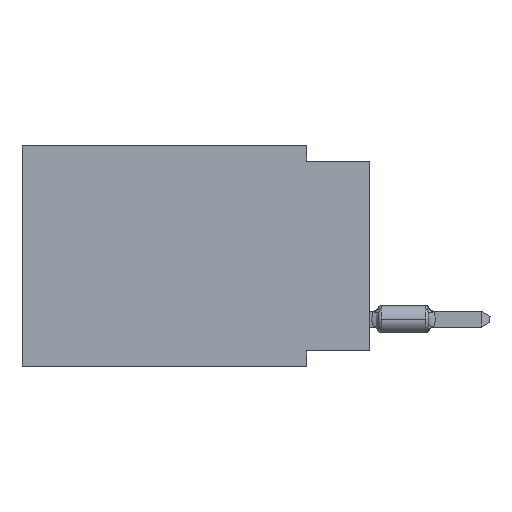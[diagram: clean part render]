
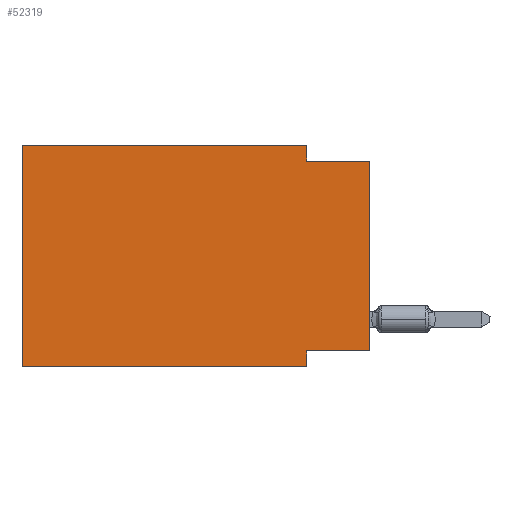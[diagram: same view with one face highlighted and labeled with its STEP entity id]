
A CAD part, left-side view. The second image highlights one B-rep face of the part: STEP entity #52319.
In plain terms, the highlighted planar face has unit normal (-1, 0, 0).
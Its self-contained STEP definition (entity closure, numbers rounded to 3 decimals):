
#66 = ORIENTED_EDGE ( 'NONE', *, *, #44495, .T. ) ;
#4127 = VERTEX_POINT ( 'NONE', #41866 ) ;
#4529 = DIRECTION ( 'NONE',  ( 0., 0., 1. ) ) ;
#5340 = CARTESIAN_POINT ( 'NONE',  ( 0., 13.97, -8.89 ) ) ;
#5358 = VECTOR ( 'NONE', #15949, 1000. ) ;
#9979 = VERTEX_POINT ( 'NONE', #30929 ) ;
#10038 = VECTOR ( 'NONE', #17574, 1000. ) ;
#10515 = VECTOR ( 'NONE', #4529, 1000. ) ;
#11270 = EDGE_CURVE ( 'NONE', #47187, #9979, #48975, .T. ) ;
#11689 = EDGE_CURVE ( 'NONE', #14714, #12453, #23586, .T. ) ;
#12295 = CARTESIAN_POINT ( 'NONE',  ( 0., 2.54, -8.89 ) ) ;
#12453 = VERTEX_POINT ( 'NONE', #47176 ) ;
#12495 = CARTESIAN_POINT ( 'NONE',  ( 0., 0., -8.255 ) ) ;
#13801 = EDGE_CURVE ( 'NONE', #48726, #14714, #18937, .T. ) ;
#14714 = VERTEX_POINT ( 'NONE', #19877 ) ;
#15577 = LINE ( 'NONE', #31042, #27015 ) ;
#15765 = CARTESIAN_POINT ( 'NONE',  ( 0., 2.54, -0.635 ) ) ;
#15949 = DIRECTION ( 'NONE',  ( 0., -1., 0. ) ) ;
#16064 = VECTOR ( 'NONE', #26564, 1000. ) ;
#17071 = VECTOR ( 'NONE', #44990, 1000. ) ;
#17255 = LINE ( 'NONE', #29495, #16064 ) ;
#17315 = LINE ( 'NONE', #33805, #10515 ) ;
#17574 = DIRECTION ( 'NONE',  ( 0., 0., -1. ) ) ;
#17610 = ORIENTED_EDGE ( 'NONE', *, *, #44813, .F. ) ;
#18937 = LINE ( 'NONE', #31460, #33401 ) ;
#19877 = CARTESIAN_POINT ( 'NONE',  ( 0., 13.97, 0. ) ) ;
#19903 = ORIENTED_EDGE ( 'NONE', *, *, #13801, .F. ) ;
#20248 = EDGE_CURVE ( 'NONE', #12453, #26433, #17255, .T. ) ;
#20904 = EDGE_CURVE ( 'NONE', #9979, #4127, #28528, .T. ) ;
#23196 = PLANE ( 'NONE',  #37482 ) ;
#23468 = CARTESIAN_POINT ( 'NONE',  ( 0., 13.97, 0. ) ) ;
#23586 = LINE ( 'NONE', #26587, #43468 ) ;
#23942 = LINE ( 'NONE', #36198, #5358 ) ;
#26433 = VERTEX_POINT ( 'NONE', #15765 ) ;
#26564 = DIRECTION ( 'NONE',  ( 0., 0., -1. ) ) ;
#26587 = CARTESIAN_POINT ( 'NONE',  ( 0., 13.97, 0. ) ) ;
#27015 = VECTOR ( 'NONE', #46735, 1000. ) ;
#27921 = ORIENTED_EDGE ( 'NONE', *, *, #20904, .F. ) ;
#28354 = ORIENTED_EDGE ( 'NONE', *, *, #11689, .F. ) ;
#28528 = LINE ( 'NONE', #12295, #10038 ) ;
#29495 = CARTESIAN_POINT ( 'NONE',  ( 0., 2.54, 0. ) ) ;
#30664 = ORIENTED_EDGE ( 'NONE', *, *, #11270, .F. ) ;
#30929 = CARTESIAN_POINT ( 'NONE',  ( 0., 2.54, -8.255 ) ) ;
#31042 = CARTESIAN_POINT ( 'NONE',  ( 0., 13.97, -8.89 ) ) ;
#31460 = CARTESIAN_POINT ( 'NONE',  ( 0., 13.97, 0. ) ) ;
#31975 = DIRECTION ( 'NONE',  ( 1., 0., 0. ) ) ;
#32531 = CARTESIAN_POINT ( 'NONE',  ( 0., 0., -0.635 ) ) ;
#33401 = VECTOR ( 'NONE', #51943, 1000. ) ;
#33805 = CARTESIAN_POINT ( 'NONE',  ( 0., 0., 0. ) ) ;
#33890 = CARTESIAN_POINT ( 'NONE',  ( 0., 0., -8.255 ) ) ;
#36198 = CARTESIAN_POINT ( 'NONE',  ( 0., 0., -0.635 ) ) ;
#36891 = EDGE_CURVE ( 'NONE', #48726, #4127, #15577, .T. ) ;
#37385 = VERTEX_POINT ( 'NONE', #32531 ) ;
#37482 = AXIS2_PLACEMENT_3D ( 'NONE', #23468, #31975, #39446 ) ;
#38371 = EDGE_LOOP ( 'NONE', ( #66, #17610, #46517, #28354, #19903, #42623, #27921, #30664 ) ) ;
#39446 = DIRECTION ( 'NONE',  ( 0., 0., -1. ) ) ;
#41866 = CARTESIAN_POINT ( 'NONE',  ( 0., 2.54, -8.89 ) ) ;
#42623 = ORIENTED_EDGE ( 'NONE', *, *, #36891, .T. ) ;
#43468 = VECTOR ( 'NONE', #52067, 1000. ) ;
#44495 = EDGE_CURVE ( 'NONE', #47187, #37385, #17315, .T. ) ;
#44813 = EDGE_CURVE ( 'NONE', #26433, #37385, #23942, .T. ) ;
#44990 = DIRECTION ( 'NONE',  ( 0., 1., 0. ) ) ;
#46517 = ORIENTED_EDGE ( 'NONE', *, *, #20248, .F. ) ;
#46735 = DIRECTION ( 'NONE',  ( 0., -1., 0. ) ) ;
#47176 = CARTESIAN_POINT ( 'NONE',  ( 0., 2.54, 0. ) ) ;
#47187 = VERTEX_POINT ( 'NONE', #33890 ) ;
#47683 = FACE_OUTER_BOUND ( 'NONE', #38371, .T. ) ;
#48726 = VERTEX_POINT ( 'NONE', #5340 ) ;
#48975 = LINE ( 'NONE', #12495, #17071 ) ;
#51943 = DIRECTION ( 'NONE',  ( 0., 0., 1. ) ) ;
#52067 = DIRECTION ( 'NONE',  ( 0., -1., 0. ) ) ;
#52319 = ADVANCED_FACE ( 'NONE', ( #47683 ), #23196, .F. ) ;
